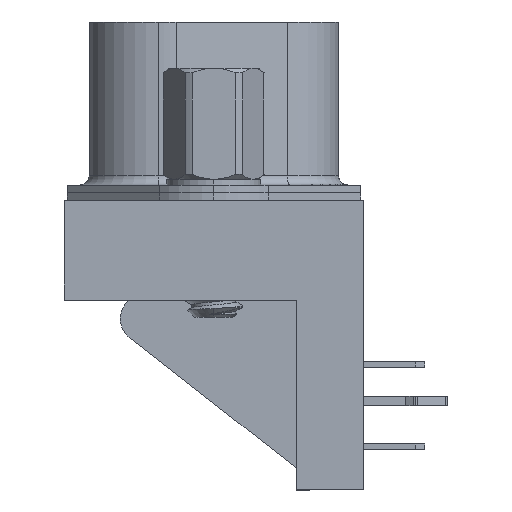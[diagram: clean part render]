
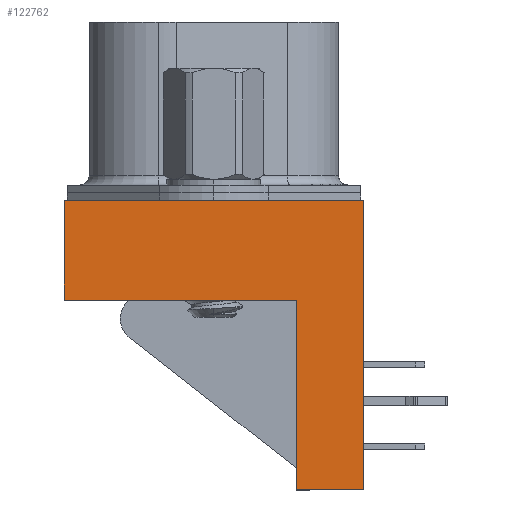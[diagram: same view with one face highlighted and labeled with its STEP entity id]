
A CAD part, left-side view. The second image highlights one B-rep face of the part: STEP entity #122762.
In plain terms, the highlighted planar face has unit normal (-1, 0, 0).
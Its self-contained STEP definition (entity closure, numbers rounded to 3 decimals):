
#3800 = EDGE_CURVE ( 'NONE', #118537, #180080, #40668, .T. ) ;
#10322 = EDGE_CURVE ( 'NONE', #60201, #90585, #24081, .T. ) ;
#12613 = VECTOR ( 'NONE', #167087, 1000. ) ;
#15413 = DIRECTION ( 'NONE',  ( 0., 0., 1. ) ) ;
#17986 = VECTOR ( 'NONE', #152813, 1000. ) ;
#22004 = CARTESIAN_POINT ( 'NONE',  ( -4.125, -7.8, -15.1 ) ) ;
#24081 = LINE ( 'NONE', #95007, #17986 ) ;
#33588 = VERTEX_POINT ( 'NONE', #114547 ) ;
#33965 = LINE ( 'NONE', #64727, #65445 ) ;
#35928 = ORIENTED_EDGE ( 'NONE', *, *, #10322, .F. ) ;
#36114 = EDGE_LOOP ( 'NONE', ( #44041, #60663, #100135, #174988, #60909, #35928 ) ) ;
#38109 = DIRECTION ( 'NONE',  ( -1., 0., 0. ) ) ;
#38612 = EDGE_CURVE ( 'NONE', #173722, #33588, #33965, .T. ) ;
#40668 = LINE ( 'NONE', #111574, #47470 ) ;
#42371 = DIRECTION ( 'NONE',  ( 0., -1., 0. ) ) ;
#44041 = ORIENTED_EDGE ( 'NONE', *, *, #96069, .F. ) ;
#45724 = CARTESIAN_POINT ( 'NONE',  ( -4.125, -4.3, -15.1 ) ) ;
#47470 = VECTOR ( 'NONE', #15413, 1000. ) ;
#50507 = EDGE_CURVE ( 'NONE', #90585, #180080, #102317, .T. ) ;
#53924 = PLANE ( 'NONE',  #138709 ) ;
#60201 = VERTEX_POINT ( 'NONE', #177307 ) ;
#60663 = ORIENTED_EDGE ( 'NONE', *, *, #38612, .F. ) ;
#60909 = ORIENTED_EDGE ( 'NONE', *, *, #50507, .F. ) ;
#64430 = CARTESIAN_POINT ( 'NONE',  ( -4.125, 7.8, 0. ) ) ;
#64727 = CARTESIAN_POINT ( 'NONE',  ( -4.125, -4.3, -15.1 ) ) ;
#64855 = LINE ( 'NONE', #126395, #109982 ) ;
#65445 = VECTOR ( 'NONE', #118898, 1000. ) ;
#81006 = CARTESIAN_POINT ( 'NONE',  ( -4.125, 7.8, -15.1 ) ) ;
#83083 = VECTOR ( 'NONE', #96391, 1000. ) ;
#90585 = VERTEX_POINT ( 'NONE', #64430 ) ;
#95007 = CARTESIAN_POINT ( 'NONE',  ( -4.125, 7.8, -15.1 ) ) ;
#96069 = EDGE_CURVE ( 'NONE', #33588, #60201, #110180, .T. ) ;
#96391 = DIRECTION ( 'NONE',  ( 0., -1., 0. ) ) ;
#100135 = ORIENTED_EDGE ( 'NONE', *, *, #136388, .T. ) ;
#102317 = LINE ( 'NONE', #178763, #83083 ) ;
#109982 = VECTOR ( 'NONE', #42371, 1000. ) ;
#110180 = LINE ( 'NONE', #179269, #12613 ) ;
#111574 = CARTESIAN_POINT ( 'NONE',  ( -4.125, -7.8, -15.1 ) ) ;
#114547 = CARTESIAN_POINT ( 'NONE',  ( -4.125, -4.3, -5.2 ) ) ;
#117543 = CARTESIAN_POINT ( 'NONE',  ( -4.125, -7.8, 0. ) ) ;
#118537 = VERTEX_POINT ( 'NONE', #22004 ) ;
#118898 = DIRECTION ( 'NONE',  ( 0., 0., 1. ) ) ;
#122762 = ADVANCED_FACE ( 'NONE', ( #137937 ), #53924, .T. ) ;
#126395 = CARTESIAN_POINT ( 'NONE',  ( -4.125, 7.8, -15.1 ) ) ;
#136388 = EDGE_CURVE ( 'NONE', #173722, #118537, #64855, .T. ) ;
#137937 = FACE_OUTER_BOUND ( 'NONE', #36114, .T. ) ;
#138709 = AXIS2_PLACEMENT_3D ( 'NONE', #81006, #38109, #179937 ) ;
#152813 = DIRECTION ( 'NONE',  ( 0., 0., 1. ) ) ;
#167087 = DIRECTION ( 'NONE',  ( 0., 1., 0. ) ) ;
#173722 = VERTEX_POINT ( 'NONE', #45724 ) ;
#174988 = ORIENTED_EDGE ( 'NONE', *, *, #3800, .T. ) ;
#177307 = CARTESIAN_POINT ( 'NONE',  ( -4.125, 7.8, -5.2 ) ) ;
#178763 = CARTESIAN_POINT ( 'NONE',  ( -4.125, 7.8, 0. ) ) ;
#179269 = CARTESIAN_POINT ( 'NONE',  ( -4.125, 7.8, -5.2 ) ) ;
#179937 = DIRECTION ( 'NONE',  ( 0., -1., 0. ) ) ;
#180080 = VERTEX_POINT ( 'NONE', #117543 ) ;
